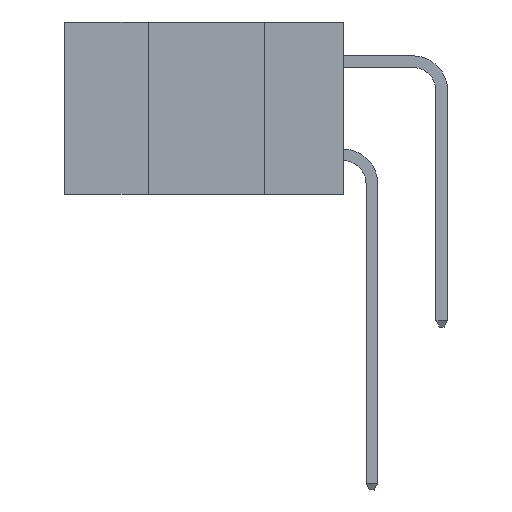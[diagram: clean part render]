
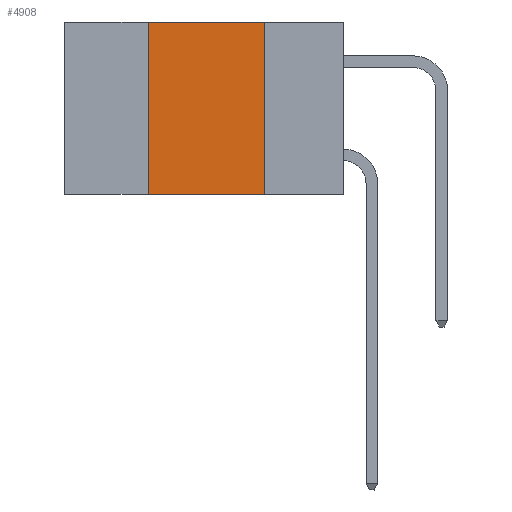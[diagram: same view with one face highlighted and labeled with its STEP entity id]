
A CAD part, left-side view. The second image highlights one B-rep face of the part: STEP entity #4908.
In plain terms, the highlighted planar face has unit normal (-1, 0, 0).
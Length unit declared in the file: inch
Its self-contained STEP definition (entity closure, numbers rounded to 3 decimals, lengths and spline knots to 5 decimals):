
#239 = VECTOR ( 'NONE', #17885, 39.37008 ) ;
#915 = LINE ( 'NONE', #4903, #20703 ) ;
#2375 = VERTEX_POINT ( 'NONE', #13552 ) ;
#3035 = CARTESIAN_POINT ( 'NONE',  ( 0., 0.42, -0.37 ) ) ;
#3269 = VERTEX_POINT ( 'NONE', #21829 ) ;
#4444 = LINE ( 'NONE', #22734, #20933 ) ;
#4903 = CARTESIAN_POINT ( 'NONE',  ( 0., 0.42, 0. ) ) ;
#4908 = ADVANCED_FACE ( 'NONE', ( #9812 ), #21246, .F. ) ;
#6570 = VERTEX_POINT ( 'NONE', #10233 ) ;
#8535 = VERTEX_POINT ( 'NONE', #3035 ) ;
#9238 = CARTESIAN_POINT ( 'NONE',  ( 0., 0.17, 0. ) ) ;
#9276 = DIRECTION ( 'NONE',  ( 0., -1., 0. ) ) ;
#9812 = FACE_OUTER_BOUND ( 'NONE', #24334, .T. ) ;
#10233 = CARTESIAN_POINT ( 'NONE',  ( 0., 0.17, -0.37 ) ) ;
#10395 = LINE ( 'NONE', #21739, #239 ) ;
#10642 = DIRECTION ( 'NONE',  ( 0., 0., 1. ) ) ;
#13552 = CARTESIAN_POINT ( 'NONE',  ( 0., 0.17, 0. ) ) ;
#13670 = LINE ( 'NONE', #9238, #23297 ) ;
#14347 = AXIS2_PLACEMENT_3D ( 'NONE', #21135, #21217, #21374 ) ;
#14526 = ORIENTED_EDGE ( 'NONE', *, *, #14651, .F. ) ;
#14651 = EDGE_CURVE ( 'NONE', #3269, #2375, #10395, .T. ) ;
#14887 = EDGE_CURVE ( 'NONE', #8535, #6570, #4444, .T. ) ;
#17885 = DIRECTION ( 'NONE',  ( 0., -1., 0. ) ) ;
#20091 = EDGE_CURVE ( 'NONE', #8535, #3269, #915, .T. ) ;
#20546 = ORIENTED_EDGE ( 'NONE', *, *, #20091, .F. ) ;
#20703 = VECTOR ( 'NONE', #10642, 39.37008 ) ;
#20933 = VECTOR ( 'NONE', #9276, 39.37008 ) ;
#21135 = CARTESIAN_POINT ( 'NONE',  ( 0., 0.6, 0. ) ) ;
#21217 = DIRECTION ( 'NONE',  ( 1., 0., 0. ) ) ;
#21246 = PLANE ( 'NONE',  #14347 ) ;
#21374 = DIRECTION ( 'NONE',  ( 0., 0., -1. ) ) ;
#21521 = EDGE_CURVE ( 'NONE', #2375, #6570, #13670, .T. ) ;
#21739 = CARTESIAN_POINT ( 'NONE',  ( 0., 0.6, 0. ) ) ;
#21829 = CARTESIAN_POINT ( 'NONE',  ( 0., 0.42, 0. ) ) ;
#22734 = CARTESIAN_POINT ( 'NONE',  ( 0., 0.6, -0.37 ) ) ;
#23297 = VECTOR ( 'NONE', #24602, 39.37008 ) ;
#23543 = ORIENTED_EDGE ( 'NONE', *, *, #21521, .F. ) ;
#24334 = EDGE_LOOP ( 'NONE', ( #23543, #14526, #20546, #24398 ) ) ;
#24398 = ORIENTED_EDGE ( 'NONE', *, *, #14887, .T. ) ;
#24602 = DIRECTION ( 'NONE',  ( 0., 0., -1. ) ) ;
